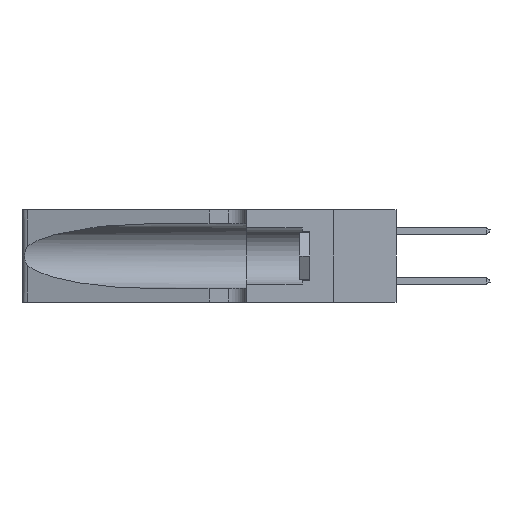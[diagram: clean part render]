
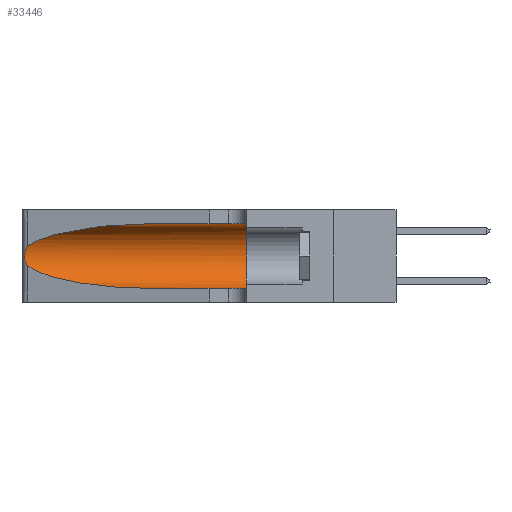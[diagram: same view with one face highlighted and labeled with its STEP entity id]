
A CAD part, left-side view. The second image highlights one B-rep face of the part: STEP entity #33446.
In plain terms, the highlighted cylindrical face has radius 3.308 mm (diameter 6.617 mm), a partial arc.
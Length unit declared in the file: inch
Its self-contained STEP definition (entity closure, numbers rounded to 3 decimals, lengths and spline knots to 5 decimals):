
#139 = DIRECTION ( 'NONE',  ( 0., 0., 1. ) ) ;
#444 = AXIS2_PLACEMENT_3D ( 'NONE', #33880, #17134, #139 ) ;
#1488 = CARTESIAN_POINT ( 'NONE',  ( 0.1305, 1.61858, 0.185 ) ) ;
#2236 = CARTESIAN_POINT ( 'NONE',  ( 0.25787, 1.23484, 0.2124 ) ) ;
#2265 = CARTESIAN_POINT ( 'NONE',  ( 0.1305, 1.61858, 0.05475 ) ) ;
#2947 = EDGE_CURVE ( 'NONE', #13133, #31620, #27520, .T. ) ;
#3355 = CARTESIAN_POINT ( 'NONE',  ( 0.25487, 1.22718, 0.14631 ) ) ;
#4368 = CARTESIAN_POINT ( 'NONE',  ( 0.1305, 0.72297, 0.31525 ) ) ;
#5100 = CARTESIAN_POINT ( 'NONE',  ( 0.26018, 1.23835, 0.19895 ) ) ;
#5125 = DIRECTION ( 'NONE',  ( 0., -1., 0. ) ) ;
#5313 = EDGE_LOOP ( 'NONE', ( #33029, #11171, #34384, #19124, #6518, #24295 ) ) ;
#6518 = ORIENTED_EDGE ( 'NONE', *, *, #33085, .F. ) ;
#7169 = DIRECTION ( 'NONE',  ( 0., -1., 0. ) ) ;
#7960 = CARTESIAN_POINT ( 'NONE',  ( 0.26075, 1.23896, 0.178 ) ) ;
#9178 = CARTESIAN_POINT ( 'NONE',  ( 0.1305, 0.35, 0.31525 ) ) ;
#9691 = CARTESIAN_POINT ( 'NONE',  ( 0.18966, 0.96281, 0.05475 ) ) ;
#10374 = CYLINDRICAL_SURFACE ( 'NONE', #28808, 0.13025 ) ;
#10824 = CARTESIAN_POINT ( 'NONE',  ( 0.25856, 1.23593, 0.16098 ) ) ;
#11003 = CARTESIAN_POINT ( 'NONE',  ( 0.1305, 0.35, 0.05475 ) ) ;
#11171 = ORIENTED_EDGE ( 'NONE', *, *, #16565, .T. ) ;
#12139 = EDGE_CURVE ( 'NONE', #25091, #28781, #12219, .T. ) ;
#12219 = LINE ( 'NONE', #24068, #34552 ) ;
#12823 = DIRECTION ( 'NONE',  ( 0., -1., 0. ) ) ;
#13133 = VERTEX_POINT ( 'NONE', #3355 ) ;
#13565 = CARTESIAN_POINT ( 'NONE',  ( 0.25487, 1.22718, 0.22369 ) ) ;
#13691 = CARTESIAN_POINT ( 'NONE',  ( 0.25639, 1.23186, 0.15144 ) ) ;
#15091 = CARTESIAN_POINT ( 'NONE',  ( 0.2373, 1.15595, 0.28018 ) ) ;
#16183 = CIRCLE ( 'NONE', #444, 0.13025 ) ;
#16535 = CARTESIAN_POINT ( 'NONE',  ( 0.25487, 1.22718, 0.14631 ) ) ;
#16565 = EDGE_CURVE ( 'NONE', #28697, #13133, #18296, .T. ) ;
#17134 = DIRECTION ( 'NONE',  ( 0., 1., 0. ) ) ;
#18296 = B_SPLINE_CURVE_WITH_KNOTS ( 'NONE', 3,
 ( #13565, #30335, #19199, #2236, #22016, #5100, #24850, #7960, #27655, #10824, #30461, #13691, #33235, #16535 ),
 .UNSPECIFIED., .F., .F.,
 ( 4, 2, 2, 2, 2, 2, 4 ),
 ( 0., 0.00027, 0.00053, 0.00107, 0.0016, 0.00187, 0.00214 ),
 .UNSPECIFIED. ) ;
#19124 = ORIENTED_EDGE ( 'NONE', *, *, #27861, .T. ) ;
#19199 = CARTESIAN_POINT ( 'NONE',  ( 0.25639, 1.23184, 0.21858 ) ) ;
#20140 = CARTESIAN_POINT ( 'NONE',  ( 0.25487, 1.22718, 0.22369 ) ) ;
#21292 = DIRECTION ( 'NONE',  ( 0., 0., -1. ) ) ;
#21974 = LINE ( 'NONE', #2265, #35957 ) ;
#22016 = CARTESIAN_POINT ( 'NONE',  ( 0.25854, 1.2359, 0.20912 ) ) ;
#24068 = CARTESIAN_POINT ( 'NONE',  ( 0.1305, 1.61858, 0.31525 ) ) ;
#24295 = ORIENTED_EDGE ( 'NONE', *, *, #12139, .F. ) ;
#24850 = CARTESIAN_POINT ( 'NONE',  ( 0.26075, 1.23896, 0.19203 ) ) ;
#25091 = VERTEX_POINT ( 'NONE', #4368 ) ;
#25331 = FACE_OUTER_BOUND ( 'NONE', #5313, .T. ) ;
#26232 = CARTESIAN_POINT ( 'NONE',  ( 0.1305, 0.72297, 0.31525 ) ) ;
#26559 = CARTESIAN_POINT ( 'NONE',  ( 0.25487, 1.22718, 0.14631 ) ) ;
#27520 =( BOUNDED_CURVE ( )  B_SPLINE_CURVE ( 3, ( #26559, #29340, #9691, #32130 ),
 .UNSPECIFIED., .F., .F. ) 
 B_SPLINE_CURVE_WITH_KNOTS ( ( 4, 4 ),
 ( 3.44316, 4.71239 ),
 .UNSPECIFIED. ) 
 CURVE ( )  GEOMETRIC_REPRESENTATION_ITEM ( )  RATIONAL_B_SPLINE_CURVE ( ( 1., 0.87, 0.87, 1. ) ) 
 REPRESENTATION_ITEM ( '' )  );
#27655 = CARTESIAN_POINT ( 'NONE',  ( 0.26017, 1.23833, 0.17102 ) ) ;
#27861 = EDGE_CURVE ( 'NONE', #31620, #30983, #21974, .T. ) ;
#28697 = VERTEX_POINT ( 'NONE', #20140 ) ;
#28781 = VERTEX_POINT ( 'NONE', #9178 ) ;
#28808 = AXIS2_PLACEMENT_3D ( 'NONE', #1488, #12823, #21292 ) ;
#29022 = CARTESIAN_POINT ( 'NONE',  ( 0.18966, 0.96281, 0.31525 ) ) ;
#29340 = CARTESIAN_POINT ( 'NONE',  ( 0.2373, 1.15595, 0.08982 ) ) ;
#30335 = CARTESIAN_POINT ( 'NONE',  ( 0.25555, 1.22994, 0.2215 ) ) ;
#30461 = CARTESIAN_POINT ( 'NONE',  ( 0.25789, 1.23486, 0.15765 ) ) ;
#30983 = VERTEX_POINT ( 'NONE', #11003 ) ;
#31620 = VERTEX_POINT ( 'NONE', #33867 ) ;
#32130 = CARTESIAN_POINT ( 'NONE',  ( 0.1305, 0.72297, 0.05475 ) ) ;
#32602 = EDGE_CURVE ( 'NONE', #25091, #28697, #35074, .T. ) ;
#33029 = ORIENTED_EDGE ( 'NONE', *, *, #32602, .T. ) ;
#33085 = EDGE_CURVE ( 'NONE', #28781, #30983, #16183, .T. ) ;
#33235 = CARTESIAN_POINT ( 'NONE',  ( 0.25555, 1.22993, 0.14849 ) ) ;
#33446 = ADVANCED_FACE ( 'NONE', ( #25331 ), #10374, .F. ) ;
#33867 = CARTESIAN_POINT ( 'NONE',  ( 0.1305, 0.72297, 0.05475 ) ) ;
#33880 = CARTESIAN_POINT ( 'NONE',  ( 0.1305, 0.35, 0.185 ) ) ;
#34384 = ORIENTED_EDGE ( 'NONE', *, *, #2947, .T. ) ;
#34552 = VECTOR ( 'NONE', #7169, 39.37008 ) ;
#34621 = CARTESIAN_POINT ( 'NONE',  ( 0.25487, 1.22718, 0.22369 ) ) ;
#35074 =( BOUNDED_CURVE ( )  B_SPLINE_CURVE ( 3, ( #26232, #29022, #15091, #34621 ),
 .UNSPECIFIED., .F., .F. ) 
 B_SPLINE_CURVE_WITH_KNOTS ( ( 4, 4 ),
 ( 1.5708, 2.84003 ),
 .UNSPECIFIED. ) 
 CURVE ( )  GEOMETRIC_REPRESENTATION_ITEM ( )  RATIONAL_B_SPLINE_CURVE ( ( 1., 0.87, 0.87, 1. ) ) 
 REPRESENTATION_ITEM ( '' )  );
#35957 = VECTOR ( 'NONE', #5125, 39.37008 ) ;
